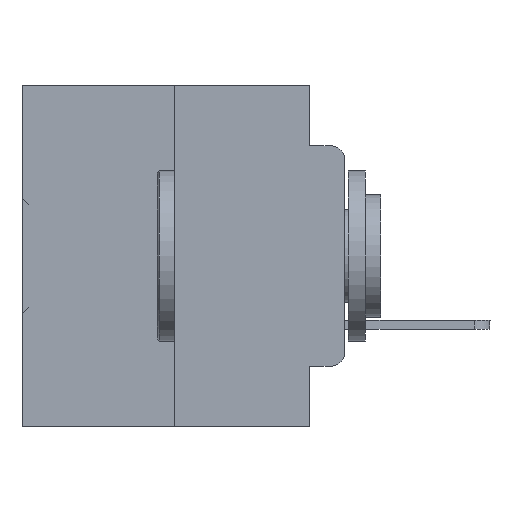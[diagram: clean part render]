
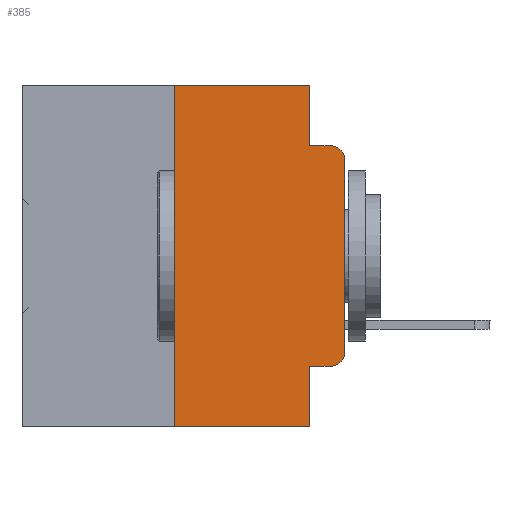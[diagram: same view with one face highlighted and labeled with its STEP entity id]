
A CAD part, left-side view. The second image highlights one B-rep face of the part: STEP entity #385.
In plain terms, the highlighted planar face has unit normal (-1, 0, 0).
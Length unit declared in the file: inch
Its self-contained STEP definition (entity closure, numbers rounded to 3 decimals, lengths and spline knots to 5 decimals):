
#385 = ADVANCED_FACE ( 'NONE', ( #22917 ), #20596, .F. ) ;
#526 = VERTEX_POINT ( 'NONE', #23565 ) ;
#2518 = VECTOR ( 'NONE', #33525, 39.37008 ) ;
#3313 = ORIENTED_EDGE ( 'NONE', *, *, #6646, .T. ) ;
#3498 = CARTESIAN_POINT ( 'NONE',  ( 0., 0.473, 0. ) ) ;
#3502 = LINE ( 'NONE', #25951, #25844 ) ;
#4082 = AXIS2_PLACEMENT_3D ( 'NONE', #3498, #23469, #9506 ) ;
#4454 = DIRECTION ( 'NONE',  ( 0., -1., 0. ) ) ;
#4750 = EDGE_CURVE ( 'NONE', #22391, #19622, #21757, .T. ) ;
#6328 = ORIENTED_EDGE ( 'NONE', *, *, #13824, .T. ) ;
#6646 = EDGE_CURVE ( 'NONE', #19622, #23775, #33650, .T. ) ;
#6980 = ORIENTED_EDGE ( 'NONE', *, *, #31822, .F. ) ;
#7427 = ORIENTED_EDGE ( 'NONE', *, *, #26242, .T. ) ;
#8242 = CARTESIAN_POINT ( 'NONE',  ( 0., 0.051, -0.4115 ) ) ;
#8289 = DIRECTION ( 'NONE',  ( 0., 0., -1. ) ) ;
#8414 = DIRECTION ( 'NONE',  ( 0., 0., -1. ) ) ;
#8715 = VECTOR ( 'NONE', #26959, 39.37008 ) ;
#8741 = AXIS2_PLACEMENT_3D ( 'NONE', #17120, #14007, #8289 ) ;
#9003 = DIRECTION ( 'NONE',  ( 0., 0., -1. ) ) ;
#9506 = DIRECTION ( 'NONE',  ( 0., 0., -1. ) ) ;
#9907 = CARTESIAN_POINT ( 'NONE',  ( 0., 0., 0. ) ) ;
#9965 = LINE ( 'NONE', #26264, #21120 ) ;
#10975 = CARTESIAN_POINT ( 'NONE',  ( 0., 0.051, 0. ) ) ;
#11114 = VECTOR ( 'NONE', #19322, 39.37008 ) ;
#11340 = VERTEX_POINT ( 'NONE', #33006 ) ;
#11682 = VERTEX_POINT ( 'NONE', #22901 ) ;
#12012 = ORIENTED_EDGE ( 'NONE', *, *, #4750, .T. ) ;
#13719 = EDGE_CURVE ( 'NONE', #29099, #16792, #25105, .T. ) ;
#13824 = EDGE_CURVE ( 'NONE', #23775, #11340, #28740, .T. ) ;
#14007 = DIRECTION ( 'NONE',  ( -1., 0., 0. ) ) ;
#15758 = CARTESIAN_POINT ( 'NONE',  ( 0., 0.051, -0.0885 ) ) ;
#16792 = VERTEX_POINT ( 'NONE', #33900 ) ;
#17120 = CARTESIAN_POINT ( 'NONE',  ( 0., 0.02, -0.3915 ) ) ;
#17145 = CARTESIAN_POINT ( 'NONE',  ( 0., 0.473, -0.5 ) ) ;
#17454 = LINE ( 'NONE', #17145, #35744 ) ;
#17554 = DIRECTION ( 'NONE',  ( 0., -1., 0. ) ) ;
#18679 = LINE ( 'NONE', #8242, #11114 ) ;
#19322 = DIRECTION ( 'NONE',  ( 0., -1., 0. ) ) ;
#19401 = ORIENTED_EDGE ( 'NONE', *, *, #36812, .F. ) ;
#19622 = VERTEX_POINT ( 'NONE', #28027 ) ;
#20269 = EDGE_CURVE ( 'NONE', #29099, #34894, #17454, .T. ) ;
#20596 = PLANE ( 'NONE',  #4082 ) ;
#20670 = ORIENTED_EDGE ( 'NONE', *, *, #20269, .T. ) ;
#21120 = VECTOR ( 'NONE', #17554, 39.37008 ) ;
#21315 = CARTESIAN_POINT ( 'NONE',  ( 0., 0.473, 0. ) ) ;
#21757 = CIRCLE ( 'NONE', #8741, 0.02 ) ;
#22098 = VECTOR ( 'NONE', #33589, 39.37008 ) ;
#22391 = VERTEX_POINT ( 'NONE', #26819 ) ;
#22623 = LINE ( 'NONE', #10975, #2518 ) ;
#22820 = LINE ( 'NONE', #21315, #29490 ) ;
#22901 = CARTESIAN_POINT ( 'NONE',  ( 0., 0.051, -0.4115 ) ) ;
#22917 = FACE_OUTER_BOUND ( 'NONE', #28971, .T. ) ;
#23469 = DIRECTION ( 'NONE',  ( 1., 0., 0. ) ) ;
#23565 = CARTESIAN_POINT ( 'NONE',  ( 0., 0.051, 0. ) ) ;
#23775 = VERTEX_POINT ( 'NONE', #24739 ) ;
#23917 = VERTEX_POINT ( 'NONE', #15758 ) ;
#24650 = ORIENTED_EDGE ( 'NONE', *, *, #29877, .F. ) ;
#24739 = CARTESIAN_POINT ( 'NONE',  ( 0., 0., -0.1085 ) ) ;
#24772 = CARTESIAN_POINT ( 'NONE',  ( 0., 0.25, -0.5 ) ) ;
#25105 = LINE ( 'NONE', #36214, #22098 ) ;
#25374 = DIRECTION ( 'NONE',  ( 0., -1., 0. ) ) ;
#25844 = VECTOR ( 'NONE', #9003, 39.37008 ) ;
#25951 = CARTESIAN_POINT ( 'NONE',  ( 0., 0.051, 0. ) ) ;
#26242 = EDGE_CURVE ( 'NONE', #11682, #22391, #18679, .T. ) ;
#26264 = CARTESIAN_POINT ( 'NONE',  ( 0., 0.051, -0.0885 ) ) ;
#26819 = CARTESIAN_POINT ( 'NONE',  ( 0., 0.02, -0.4115 ) ) ;
#26959 = DIRECTION ( 'NONE',  ( 0., 0., 1. ) ) ;
#28027 = CARTESIAN_POINT ( 'NONE',  ( 0., 0., -0.3915 ) ) ;
#28740 = CIRCLE ( 'NONE', #29700, 0.02 ) ;
#28971 = EDGE_LOOP ( 'NONE', ( #3313, #6328, #6980, #24650, #19401, #32169, #20670, #36149, #7427, #12012 ) ) ;
#29099 = VERTEX_POINT ( 'NONE', #24772 ) ;
#29490 = VECTOR ( 'NONE', #4454, 39.37008 ) ;
#29700 = AXIS2_PLACEMENT_3D ( 'NONE', #33842, #36965, #8414 ) ;
#29877 = EDGE_CURVE ( 'NONE', #526, #23917, #22623, .T. ) ;
#31642 = CARTESIAN_POINT ( 'NONE',  ( 0., 0.051, -0.5 ) ) ;
#31822 = EDGE_CURVE ( 'NONE', #23917, #11340, #9965, .T. ) ;
#32169 = ORIENTED_EDGE ( 'NONE', *, *, #13719, .F. ) ;
#33006 = CARTESIAN_POINT ( 'NONE',  ( 0., 0.02, -0.0885 ) ) ;
#33525 = DIRECTION ( 'NONE',  ( 0., 0., -1. ) ) ;
#33589 = DIRECTION ( 'NONE',  ( 0., 0., 1. ) ) ;
#33650 = LINE ( 'NONE', #9907, #8715 ) ;
#33842 = CARTESIAN_POINT ( 'NONE',  ( 0., 0.02, -0.1085 ) ) ;
#33900 = CARTESIAN_POINT ( 'NONE',  ( 0., 0.25, 0. ) ) ;
#34231 = EDGE_CURVE ( 'NONE', #11682, #34894, #3502, .T. ) ;
#34894 = VERTEX_POINT ( 'NONE', #31642 ) ;
#35744 = VECTOR ( 'NONE', #25374, 39.37008 ) ;
#36149 = ORIENTED_EDGE ( 'NONE', *, *, #34231, .F. ) ;
#36214 = CARTESIAN_POINT ( 'NONE',  ( 0., 0.25, 0. ) ) ;
#36812 = EDGE_CURVE ( 'NONE', #16792, #526, #22820, .T. ) ;
#36965 = DIRECTION ( 'NONE',  ( -1., 0., 0. ) ) ;
